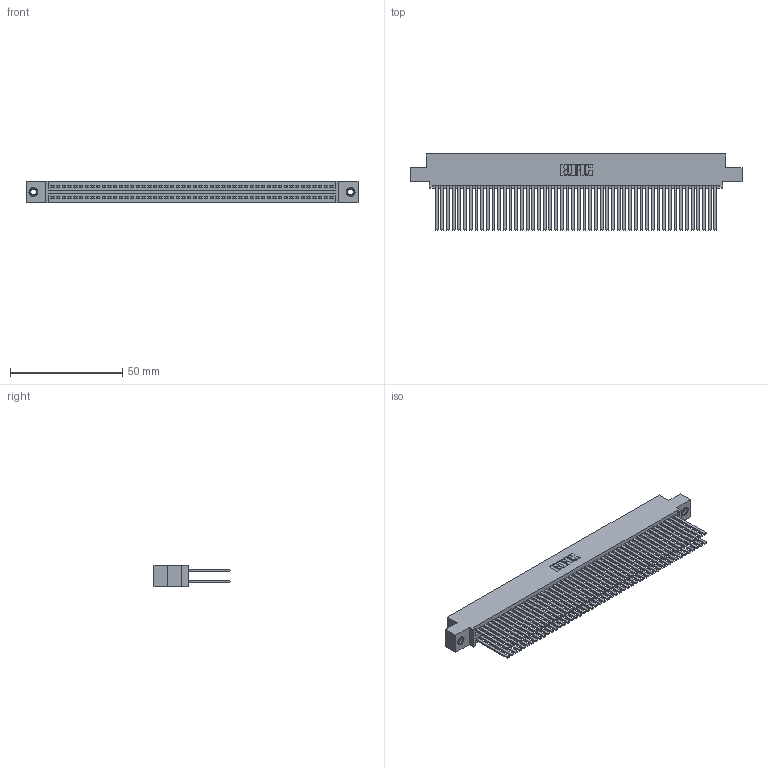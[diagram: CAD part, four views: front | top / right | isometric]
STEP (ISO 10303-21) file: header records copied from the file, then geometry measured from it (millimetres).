
FILE_DESCRIPTION (( 'STEP AP203' ), '1' );
FILE_NAME ('395-100-544-507.STEP', '2018-11-30T02:31:38', ( '' ), ( '' ), 'SwSTEP 2.0', 'SolidWorks 2016', '' );
FILE_SCHEMA (( 'CONFIG_CONTROL_DESIGN' ));
Length unit declared in the file: inch
Products named in the file (4): 345 Part_0.110 Offset - 0.156 Dia-TI; 395-100-544-507; 345-292-001_345-293-144; 345-250-001_345-250-005-103
Assembly tree (103 placements, depth 2):
  395-100-544-507
    345 Part_0.110 Offset - 0.156 Dia-TI
    345-292-001_345-293-144  x100
    345-250-001_345-250-005-103  x2
Bounding box: 148.21 x 33.96 x 9.4 mm (x, y, z)
Volume: 15786.4 mm3; surface area: 27719.2 mm2
Topology: 103 solids, 103 shells, 4590 faces, 13589 edges, 8918 vertices
Faces by surface type: plane 3016, cylinder 1558, cone 12, torus 4
Entity records: 39288 total; most frequent: CARTESIAN_POINT 6559, ORIENTED_EDGE 6486, DIRECTION 5797, EDGE_CURVE 3243, LINE 2895, VECTOR 2895, VERTEX_POINT 2156, AXIS2_PLACEMENT_3D 1451
